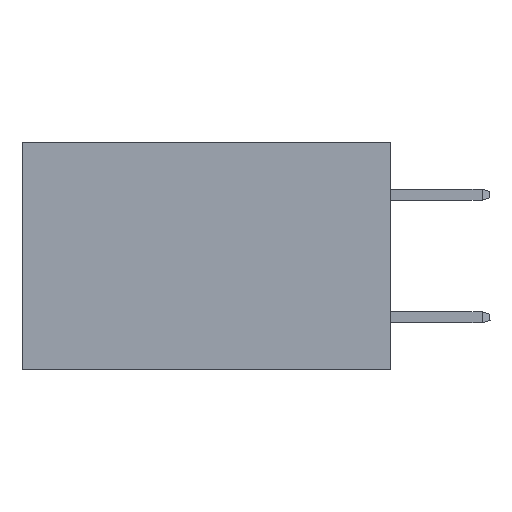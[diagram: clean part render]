
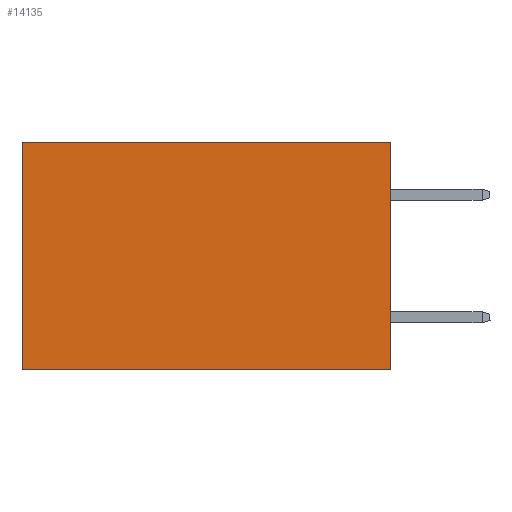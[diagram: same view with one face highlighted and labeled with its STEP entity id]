
A CAD part, left-side view. The second image highlights one B-rep face of the part: STEP entity #14135.
In plain terms, the highlighted planar face has unit normal (-1, 0, 0).
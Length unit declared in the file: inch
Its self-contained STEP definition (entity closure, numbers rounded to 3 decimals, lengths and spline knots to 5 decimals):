
#30 = VERTEX_POINT ( 'NONE', #11778 ) ;
#1201 = LINE ( 'NONE', #30034, #3176 ) ;
#1773 = VERTEX_POINT ( 'NONE', #19649 ) ;
#1945 = VERTEX_POINT ( 'NONE', #2610 ) ;
#1955 = DIRECTION ( 'NONE',  ( 0., 0., -1. ) ) ;
#2198 = CARTESIAN_POINT ( 'NONE',  ( 0.2875, 0., -0.37 ) ) ;
#2610 = CARTESIAN_POINT ( 'NONE',  ( 0.2875, 0.6, 0. ) ) ;
#3176 = VECTOR ( 'NONE', #27558, 39.37008 ) ;
#3800 = VECTOR ( 'NONE', #17294, 39.37008 ) ;
#4001 = VERTEX_POINT ( 'NONE', #11808 ) ;
#5195 = ORIENTED_EDGE ( 'NONE', *, *, #8310, .T. ) ;
#7975 = VECTOR ( 'NONE', #18212, 39.37008 ) ;
#8310 = EDGE_CURVE ( 'NONE', #1773, #1945, #20713, .T. ) ;
#9932 = LINE ( 'NONE', #10449, #7975 ) ;
#10217 = EDGE_CURVE ( 'NONE', #30, #4001, #17404, .T. ) ;
#10449 = CARTESIAN_POINT ( 'NONE',  ( 0.2875, 0.6, 0. ) ) ;
#11778 = CARTESIAN_POINT ( 'NONE',  ( 0.2875, 0., -0.37 ) ) ;
#11808 = CARTESIAN_POINT ( 'NONE',  ( 0.2875, 0.6, -0.37 ) ) ;
#14135 = ADVANCED_FACE ( 'NONE', ( #28728 ), #16732, .F. ) ;
#16732 = PLANE ( 'NONE',  #22127 ) ;
#16847 = DIRECTION ( 'NONE',  ( 1., 0., 0. ) ) ;
#17294 = DIRECTION ( 'NONE',  ( 0., 1., 0. ) ) ;
#17404 = LINE ( 'NONE', #2198, #3800 ) ;
#17619 = ORIENTED_EDGE ( 'NONE', *, *, #10217, .F. ) ;
#18212 = DIRECTION ( 'NONE',  ( 0., 0., -1. ) ) ;
#18378 = EDGE_CURVE ( 'NONE', #1773, #30, #1201, .T. ) ;
#19542 = CARTESIAN_POINT ( 'NONE',  ( 0.2875, 0., 0. ) ) ;
#19649 = CARTESIAN_POINT ( 'NONE',  ( 0.2875, 0., 0. ) ) ;
#20713 = LINE ( 'NONE', #21871, #31923 ) ;
#21871 = CARTESIAN_POINT ( 'NONE',  ( 0.2875, 0., 0. ) ) ;
#22127 = AXIS2_PLACEMENT_3D ( 'NONE', #19542, #16847, #1955 ) ;
#22173 = EDGE_CURVE ( 'NONE', #1945, #4001, #9932, .T. ) ;
#26949 = ORIENTED_EDGE ( 'NONE', *, *, #22173, .T. ) ;
#27558 = DIRECTION ( 'NONE',  ( 0., 0., -1. ) ) ;
#28728 = FACE_OUTER_BOUND ( 'NONE', #30036, .T. ) ;
#29558 = DIRECTION ( 'NONE',  ( 0., 1., 0. ) ) ;
#30034 = CARTESIAN_POINT ( 'NONE',  ( 0.2875, 0., 0. ) ) ;
#30036 = EDGE_LOOP ( 'NONE', ( #26949, #17619, #30408, #5195 ) ) ;
#30408 = ORIENTED_EDGE ( 'NONE', *, *, #18378, .F. ) ;
#31923 = VECTOR ( 'NONE', #29558, 39.37008 ) ;
